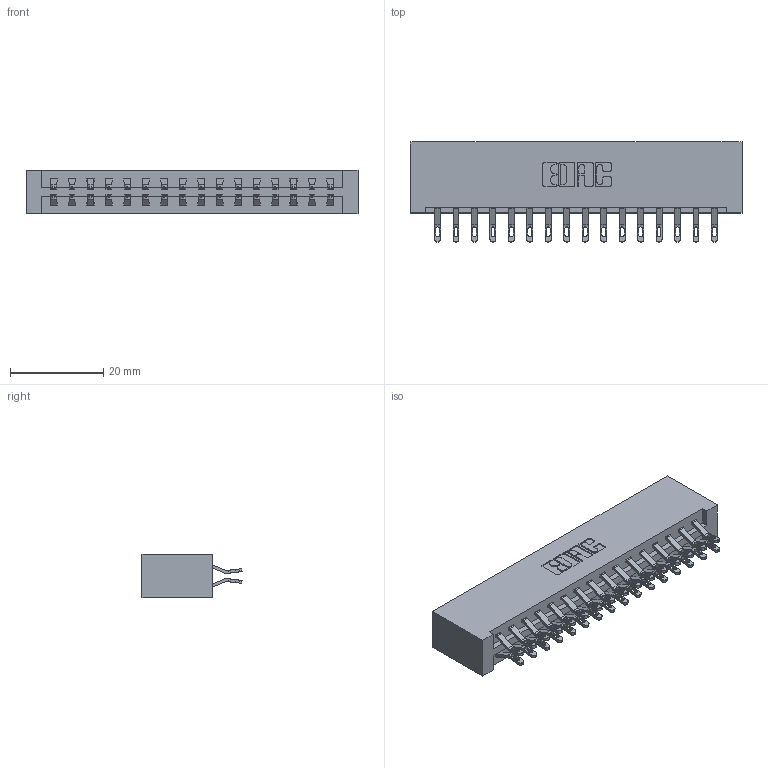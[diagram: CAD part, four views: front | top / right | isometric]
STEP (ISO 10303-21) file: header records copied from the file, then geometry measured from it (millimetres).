
FILE_DESCRIPTION (( 'STEP AP203' ), '1' );
FILE_NAME ('337-032-555-201.STEP', '2018-08-07T06:48:51', ( '' ), ( '' ), 'SwSTEP 2.0', 'SolidWorks 2016', '' );
FILE_SCHEMA (( 'CONFIG_CONTROL_DESIGN' ));
Length unit declared in the file: inch
Products named in the file (3): 337 Part_No Mounting Lugs; 345-292-001_555 Tail; 337-032-555-201
Assembly tree (33 placements, depth 2):
  337-032-555-201
    337 Part_No Mounting Lugs
    345-292-001_555 Tail  x32
Bounding box: 71.27 x 21.47 x 9.4 mm (x, y, z)
Volume: 8018.7 mm3; surface area: 9218.5 mm2
Topology: 33 solids, 33 shells, 2026 faces, 6335 edges, 4222 vertices
Faces by surface type: plane 1218, cylinder 808
Entity records: 15817 total; most frequent: CARTESIAN_POINT 2720, ORIENTED_EDGE 2626, DIRECTION 2325, EDGE_CURVE 1313, LINE 1173, VECTOR 1173, VERTEX_POINT 874, AXIS2_PLACEMENT_3D 576
